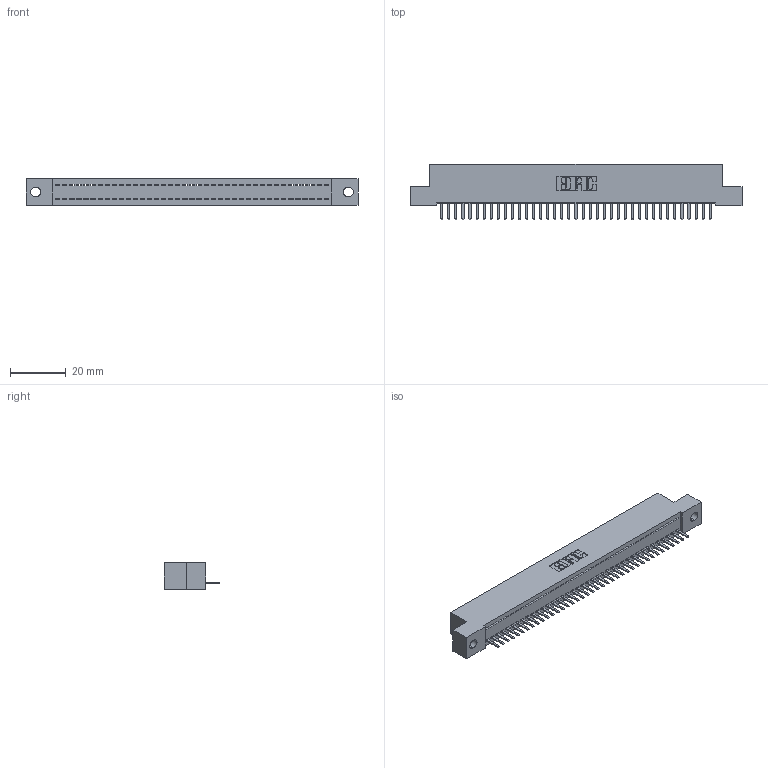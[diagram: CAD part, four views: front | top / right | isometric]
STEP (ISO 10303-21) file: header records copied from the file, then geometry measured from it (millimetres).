
FILE_DESCRIPTION (( 'STEP AP203' ), '1' );
FILE_NAME ('392-039-520-102.STEP', '2018-08-16T06:10:05', ( '' ), ( '' ), 'SwSTEP 2.0', 'SolidWorks 2016', '' );
FILE_SCHEMA (( 'CONFIG_CONTROL_DESIGN' ));
Length unit declared in the file: inch
Products named in the file (3): 342 Part_.128 Slot; 345-292-001_345-293-120; 392-039-520-102
Assembly tree (40 placements, depth 2):
  392-039-520-102
    342 Part_.128 Slot
    345-292-001_345-293-120  x39
Bounding box: 119.38 x 20.02 x 9.4 mm (x, y, z)
Volume: 10291.9 mm3; surface area: 14458 mm2
Topology: 40 solids, 40 shells, 2532 faces, 7487 edges, 4886 vertices
Faces by surface type: plane 1786, cylinder 746
Entity records: 24347 total; most frequent: CARTESIAN_POINT 4219, ORIENTED_EDGE 4182, DIRECTION 3553, EDGE_CURVE 2091, VECTOR 1959, LINE 1959, VERTEX_POINT 1390, AXIS2_PLACEMENT_3D 797
